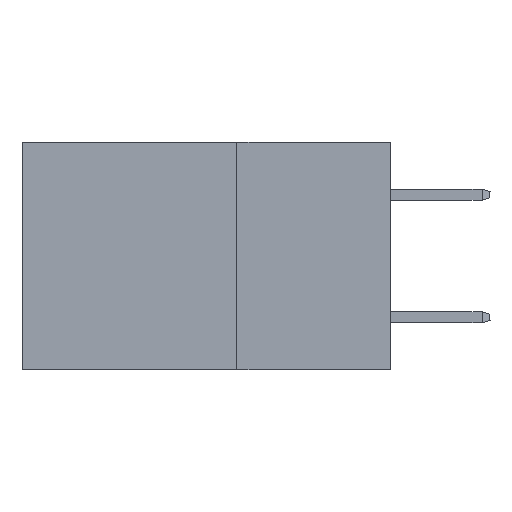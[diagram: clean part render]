
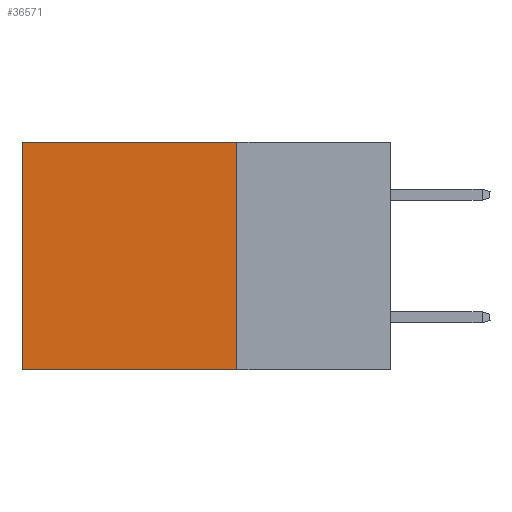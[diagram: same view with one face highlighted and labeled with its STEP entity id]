
A CAD part, left-side view. The second image highlights one B-rep face of the part: STEP entity #36571.
In plain terms, the highlighted planar face has unit normal (-1, 0, 0).
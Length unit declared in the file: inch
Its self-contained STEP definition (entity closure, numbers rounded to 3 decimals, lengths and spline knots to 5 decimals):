
#3266 = VECTOR ( 'NONE', #15720, 39.37008 ) ;
#3540 = DIRECTION ( 'NONE',  ( 0., 0., -1. ) ) ;
#4934 = VERTEX_POINT ( 'NONE', #36689 ) ;
#7241 = VERTEX_POINT ( 'NONE', #26484 ) ;
#7449 = LINE ( 'NONE', #33546, #34515 ) ;
#9210 = EDGE_CURVE ( 'NONE', #7241, #4934, #18680, .T. ) ;
#11621 = CARTESIAN_POINT ( 'NONE',  ( 0.2875, 0.6, -0.37 ) ) ;
#12830 = CARTESIAN_POINT ( 'NONE',  ( 0.2875, 0.25, 0. ) ) ;
#13016 = VECTOR ( 'NONE', #30269, 39.37008 ) ;
#14467 = EDGE_CURVE ( 'NONE', #4934, #17925, #7449, .T. ) ;
#14615 = LINE ( 'NONE', #32410, #26826 ) ;
#14934 = CARTESIAN_POINT ( 'NONE',  ( 0.2875, 0.25, 0. ) ) ;
#15720 = DIRECTION ( 'NONE',  ( 0., 0., -1. ) ) ;
#17598 = EDGE_CURVE ( 'NONE', #7241, #25826, #14615, .T. ) ;
#17714 = PLANE ( 'NONE',  #24473 ) ;
#17925 = VERTEX_POINT ( 'NONE', #11621 ) ;
#18680 = LINE ( 'NONE', #12830, #3266 ) ;
#20612 = EDGE_LOOP ( 'NONE', ( #25233, #34613, #26359, #35837 ) ) ;
#20863 = DIRECTION ( 'NONE',  ( 1., 0., 0. ) ) ;
#21291 = CARTESIAN_POINT ( 'NONE',  ( 0.2875, 0.6, 0. ) ) ;
#24473 = AXIS2_PLACEMENT_3D ( 'NONE', #14934, #20863, #3540 ) ;
#25233 = ORIENTED_EDGE ( 'NONE', *, *, #28554, .T. ) ;
#25826 = VERTEX_POINT ( 'NONE', #35831 ) ;
#26359 = ORIENTED_EDGE ( 'NONE', *, *, #9210, .F. ) ;
#26484 = CARTESIAN_POINT ( 'NONE',  ( 0.2875, 0.25, 0. ) ) ;
#26826 = VECTOR ( 'NONE', #26869, 39.37008 ) ;
#26869 = DIRECTION ( 'NONE',  ( 0., 1., 0. ) ) ;
#27466 = LINE ( 'NONE', #21291, #13016 ) ;
#28554 = EDGE_CURVE ( 'NONE', #25826, #17925, #27466, .T. ) ;
#29047 = FACE_OUTER_BOUND ( 'NONE', #20612, .T. ) ;
#30269 = DIRECTION ( 'NONE',  ( 0., 0., -1. ) ) ;
#32410 = CARTESIAN_POINT ( 'NONE',  ( 0.2875, 0.25, 0. ) ) ;
#33546 = CARTESIAN_POINT ( 'NONE',  ( 0.2875, 0.25, -0.37 ) ) ;
#34515 = VECTOR ( 'NONE', #36574, 39.37008 ) ;
#34613 = ORIENTED_EDGE ( 'NONE', *, *, #14467, .F. ) ;
#35831 = CARTESIAN_POINT ( 'NONE',  ( 0.2875, 0.6, 0. ) ) ;
#35837 = ORIENTED_EDGE ( 'NONE', *, *, #17598, .T. ) ;
#36571 = ADVANCED_FACE ( 'NONE', ( #29047 ), #17714, .F. ) ;
#36574 = DIRECTION ( 'NONE',  ( 0., 1., 0. ) ) ;
#36689 = CARTESIAN_POINT ( 'NONE',  ( 0.2875, 0.25, -0.37 ) ) ;
